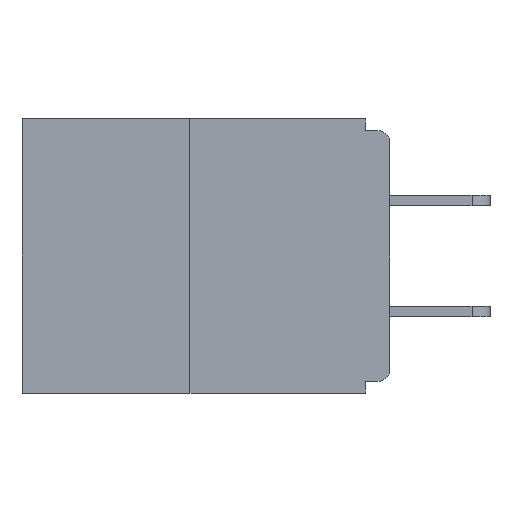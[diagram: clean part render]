
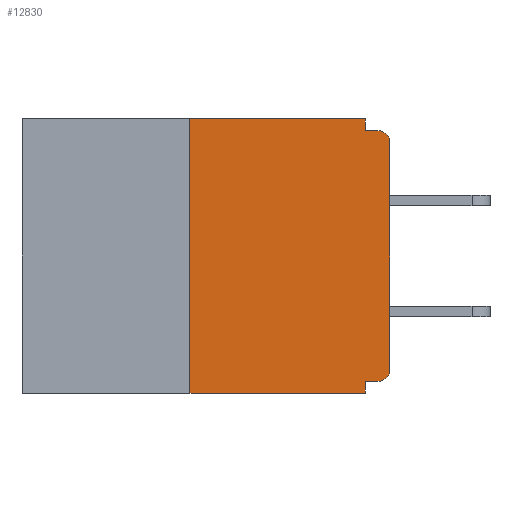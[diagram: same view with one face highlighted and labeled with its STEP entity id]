
A CAD part, left-side view. The second image highlights one B-rep face of the part: STEP entity #12830.
In plain terms, the highlighted planar face has unit normal (-1, 0, 0).
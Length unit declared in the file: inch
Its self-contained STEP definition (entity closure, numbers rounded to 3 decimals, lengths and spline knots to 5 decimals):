
#220 = CARTESIAN_POINT ( 'NONE',  ( 0., 0.031, -0.328 ) ) ;
#230 = PLANE ( 'NONE',  #16285 ) ;
#849 = CARTESIAN_POINT ( 'NONE',  ( 0., 0.015, -0.313 ) ) ;
#854 = CARTESIAN_POINT ( 'NONE',  ( 0., 0.031, 0. ) ) ;
#1480 = VERTEX_POINT ( 'NONE', #19331 ) ;
#1981 = VERTEX_POINT ( 'NONE', #18977 ) ;
#2054 = DIRECTION ( 'NONE',  ( 0., 0., -1. ) ) ;
#2220 = EDGE_CURVE ( 'NONE', #1981, #20805, #3649, .T. ) ;
#2462 = VECTOR ( 'NONE', #2054, 39.37008 ) ;
#2751 = VECTOR ( 'NONE', #19531, 39.37008 ) ;
#3277 = LINE ( 'NONE', #854, #6675 ) ;
#3497 = CARTESIAN_POINT ( 'NONE',  ( 0., 0.031, 0. ) ) ;
#3626 = VERTEX_POINT ( 'NONE', #13092 ) ;
#3649 = LINE ( 'NONE', #6230, #20279 ) ;
#4605 = CARTESIAN_POINT ( 'NONE',  ( 0., 0.015, -0.03 ) ) ;
#4774 = VERTEX_POINT ( 'NONE', #16495 ) ;
#4891 = ORIENTED_EDGE ( 'NONE', *, *, #30785, .T. ) ;
#5086 = CARTESIAN_POINT ( 'NONE',  ( 0., 0.46, 0. ) ) ;
#5767 = EDGE_LOOP ( 'NONE', ( #14688, #10540, #29428, #26623, #8171, #29062, #30030, #4891, #16263, #5884 ) ) ;
#5884 = ORIENTED_EDGE ( 'NONE', *, *, #13477, .F. ) ;
#6230 = CARTESIAN_POINT ( 'NONE',  ( 0., 0., -0.328 ) ) ;
#6675 = VECTOR ( 'NONE', #8480, 39.37008 ) ;
#7247 = VERTEX_POINT ( 'NONE', #11543 ) ;
#7770 = VECTOR ( 'NONE', #11497, 39.37008 ) ;
#7893 = DIRECTION ( 'NONE',  ( 0., -1., 0. ) ) ;
#8171 = ORIENTED_EDGE ( 'NONE', *, *, #2220, .F. ) ;
#8267 = DIRECTION ( 'NONE',  ( 0., 0., -1. ) ) ;
#8270 = LINE ( 'NONE', #12617, #22577 ) ;
#8480 = DIRECTION ( 'NONE',  ( 0., 0., -1. ) ) ;
#10112 = VECTOR ( 'NONE', #21488, 39.37008 ) ;
#10363 = CARTESIAN_POINT ( 'NONE',  ( 0., 0.031, -0.015 ) ) ;
#10540 = ORIENTED_EDGE ( 'NONE', *, *, #11329, .F. ) ;
#10856 = EDGE_CURVE ( 'NONE', #3626, #13051, #8270, .T. ) ;
#11329 = EDGE_CURVE ( 'NONE', #25530, #3626, #30387, .T. ) ;
#11497 = DIRECTION ( 'NONE',  ( 0., -1., 0. ) ) ;
#11543 = CARTESIAN_POINT ( 'NONE',  ( 0., 0.015, -0.015 ) ) ;
#12053 = AXIS2_PLACEMENT_3D ( 'NONE', #4605, #21474, #21059 ) ;
#12617 = CARTESIAN_POINT ( 'NONE',  ( 0., 0.46, 0. ) ) ;
#12830 = ADVANCED_FACE ( 'NONE', ( #22052 ), #230, .F. ) ;
#13051 = VERTEX_POINT ( 'NONE', #3497 ) ;
#13092 = CARTESIAN_POINT ( 'NONE',  ( 0., 0.25, 0. ) ) ;
#13477 = EDGE_CURVE ( 'NONE', #13051, #30630, #3277, .T. ) ;
#13484 = DIRECTION ( 'NONE',  ( 0., 1., 0. ) ) ;
#14688 = ORIENTED_EDGE ( 'NONE', *, *, #10856, .F. ) ;
#15893 = CIRCLE ( 'NONE', #12053, 0.015 ) ;
#16040 = EDGE_CURVE ( 'NONE', #1480, #4774, #28098, .T. ) ;
#16263 = ORIENTED_EDGE ( 'NONE', *, *, #19405, .F. ) ;
#16285 = AXIS2_PLACEMENT_3D ( 'NONE', #5086, #26762, #29138 ) ;
#16495 = CARTESIAN_POINT ( 'NONE',  ( 0., 0., -0.03 ) ) ;
#16625 = CARTESIAN_POINT ( 'NONE',  ( 0., 0.25, 0. ) ) ;
#16876 = AXIS2_PLACEMENT_3D ( 'NONE', #849, #25072, #8267 ) ;
#18977 = CARTESIAN_POINT ( 'NONE',  ( 0., 0.015, -0.328 ) ) ;
#19331 = CARTESIAN_POINT ( 'NONE',  ( 0., 0., -0.313 ) ) ;
#19405 = EDGE_CURVE ( 'NONE', #30630, #7247, #28684, .T. ) ;
#19531 = DIRECTION ( 'NONE',  ( 0., -1., 0. ) ) ;
#19829 = EDGE_CURVE ( 'NONE', #25530, #23229, #29167, .T. ) ;
#20279 = VECTOR ( 'NONE', #13484, 39.37008 ) ;
#20805 = VERTEX_POINT ( 'NONE', #220 ) ;
#20889 = CARTESIAN_POINT ( 'NONE',  ( 0., 0.031, -0.343 ) ) ;
#21059 = DIRECTION ( 'NONE',  ( 0., 0., -1. ) ) ;
#21157 = CARTESIAN_POINT ( 'NONE',  ( 0., 0.25, -0.343 ) ) ;
#21474 = DIRECTION ( 'NONE',  ( -1., 0., 0. ) ) ;
#21488 = DIRECTION ( 'NONE',  ( 0., 0., 1. ) ) ;
#21897 = CARTESIAN_POINT ( 'NONE',  ( 0., 0., 0. ) ) ;
#22052 = FACE_OUTER_BOUND ( 'NONE', #5767, .T. ) ;
#22577 = VECTOR ( 'NONE', #7893, 39.37008 ) ;
#23079 = EDGE_CURVE ( 'NONE', #1981, #1480, #30219, .T. ) ;
#23229 = VERTEX_POINT ( 'NONE', #20889 ) ;
#24057 = VECTOR ( 'NONE', #31092, 39.37008 ) ;
#24332 = CARTESIAN_POINT ( 'NONE',  ( 0., 0., -0.015 ) ) ;
#25072 = DIRECTION ( 'NONE',  ( -1., 0., 0. ) ) ;
#25530 = VERTEX_POINT ( 'NONE', #21157 ) ;
#25936 = CARTESIAN_POINT ( 'NONE',  ( 0., 0.031, -0.343 ) ) ;
#26107 = CARTESIAN_POINT ( 'NONE',  ( 0., 0.46, -0.343 ) ) ;
#26192 = EDGE_CURVE ( 'NONE', #20805, #23229, #29512, .T. ) ;
#26623 = ORIENTED_EDGE ( 'NONE', *, *, #26192, .F. ) ;
#26762 = DIRECTION ( 'NONE',  ( 1., 0., 0. ) ) ;
#28098 = LINE ( 'NONE', #21897, #10112 ) ;
#28684 = LINE ( 'NONE', #24332, #2751 ) ;
#29062 = ORIENTED_EDGE ( 'NONE', *, *, #23079, .T. ) ;
#29138 = DIRECTION ( 'NONE',  ( 0., 0., -1. ) ) ;
#29167 = LINE ( 'NONE', #26107, #7770 ) ;
#29428 = ORIENTED_EDGE ( 'NONE', *, *, #19829, .T. ) ;
#29512 = LINE ( 'NONE', #25936, #2462 ) ;
#30030 = ORIENTED_EDGE ( 'NONE', *, *, #16040, .T. ) ;
#30219 = CIRCLE ( 'NONE', #16876, 0.015 ) ;
#30387 = LINE ( 'NONE', #16625, #24057 ) ;
#30630 = VERTEX_POINT ( 'NONE', #10363 ) ;
#30785 = EDGE_CURVE ( 'NONE', #4774, #7247, #15893, .T. ) ;
#31092 = DIRECTION ( 'NONE',  ( 0., 0., 1. ) ) ;
